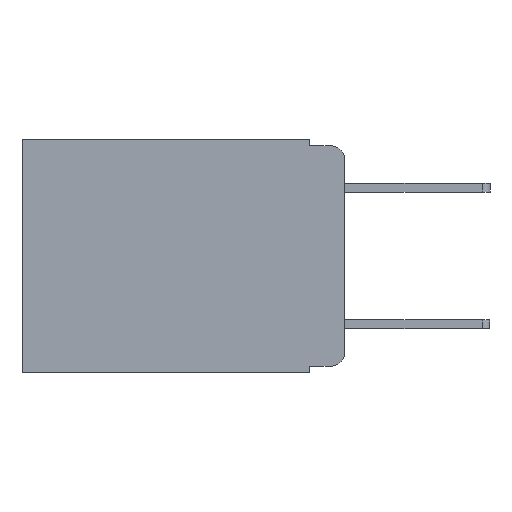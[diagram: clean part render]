
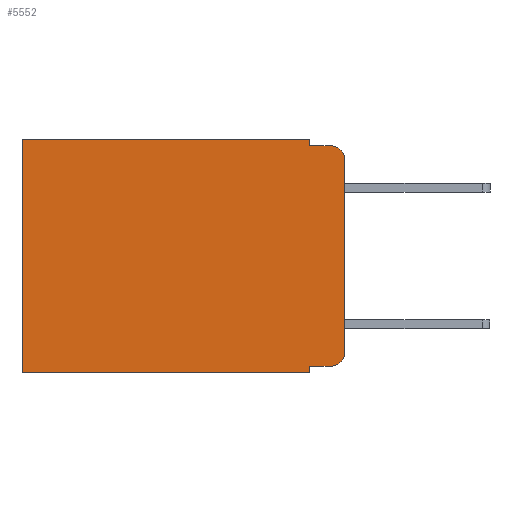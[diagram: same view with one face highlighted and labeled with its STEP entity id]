
A CAD part, left-side view. The second image highlights one B-rep face of the part: STEP entity #5552.
In plain terms, the highlighted planar face has unit normal (-1, 0, 0).
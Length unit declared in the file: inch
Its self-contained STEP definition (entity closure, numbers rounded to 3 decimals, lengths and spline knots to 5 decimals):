
#8 = VECTOR ( 'NONE', #10532, 39.37008 ) ;
#55 = CARTESIAN_POINT ( 'NONE',  ( 0.298, 0., 0. ) ) ;
#205 = LINE ( 'NONE', #9611, #5997 ) ;
#287 = ORIENTED_EDGE ( 'NONE', *, *, #2690, .F. ) ;
#311 = CARTESIAN_POINT ( 'NONE',  ( 0.298, 0.02, -0.333 ) ) ;
#372 = VECTOR ( 'NONE', #2864, 39.37008 ) ;
#613 = VERTEX_POINT ( 'NONE', #10655 ) ;
#626 = ORIENTED_EDGE ( 'NONE', *, *, #2716, .T. ) ;
#729 = CARTESIAN_POINT ( 'NONE',  ( 0.298, 0.473, 0. ) ) ;
#825 = ORIENTED_EDGE ( 'NONE', *, *, #6693, .T. ) ;
#1047 = LINE ( 'NONE', #729, #372 ) ;
#1069 = VERTEX_POINT ( 'NONE', #9491 ) ;
#1205 = VECTOR ( 'NONE', #4207, 39.37008 ) ;
#1219 = DIRECTION ( 'NONE',  ( 1., 0., 0. ) ) ;
#1309 = AXIS2_PLACEMENT_3D ( 'NONE', #1734, #8865, #2820 ) ;
#1691 = ORIENTED_EDGE ( 'NONE', *, *, #2676, .F. ) ;
#1734 = CARTESIAN_POINT ( 'NONE',  ( 0.298, 0.02, -0.03 ) ) ;
#1859 = CARTESIAN_POINT ( 'NONE',  ( 0.298, 0., -0.03 ) ) ;
#1904 = ORIENTED_EDGE ( 'NONE', *, *, #8988, .F. ) ;
#2116 = ORIENTED_EDGE ( 'NONE', *, *, #6798, .F. ) ;
#2216 = EDGE_LOOP ( 'NONE', ( #1904, #2267, #287, #1691, #626, #825, #2370, #2116, #2641, #12103 ) ) ;
#2230 = VERTEX_POINT ( 'NONE', #11432 ) ;
#2267 = ORIENTED_EDGE ( 'NONE', *, *, #8161, .T. ) ;
#2370 = ORIENTED_EDGE ( 'NONE', *, *, #3287, .F. ) ;
#2606 = DIRECTION ( 'NONE',  ( 0., -1., 0. ) ) ;
#2641 = ORIENTED_EDGE ( 'NONE', *, *, #7131, .T. ) ;
#2676 = EDGE_CURVE ( 'NONE', #1069, #2230, #3109, .T. ) ;
#2690 = EDGE_CURVE ( 'NONE', #2230, #613, #11928, .T. ) ;
#2716 = EDGE_CURVE ( 'NONE', #1069, #6191, #8904, .T. ) ;
#2820 = DIRECTION ( 'NONE',  ( 0., 0., -1. ) ) ;
#2864 = DIRECTION ( 'NONE',  ( 0., 0., -1. ) ) ;
#3109 = LINE ( 'NONE', #11004, #4253 ) ;
#3244 = LINE ( 'NONE', #5622, #8 ) ;
#3287 = EDGE_CURVE ( 'NONE', #9546, #12677, #205, .T. ) ;
#3580 = VECTOR ( 'NONE', #7004, 39.37008 ) ;
#3640 = VERTEX_POINT ( 'NONE', #10193 ) ;
#3723 = CARTESIAN_POINT ( 'NONE',  ( 0.298, 0.02, -0.313 ) ) ;
#4207 = DIRECTION ( 'NONE',  ( 0., 0., -1. ) ) ;
#4253 = VECTOR ( 'NONE', #11816, 39.37008 ) ;
#4535 = VECTOR ( 'NONE', #8374, 39.37008 ) ;
#4757 = DIRECTION ( 'NONE',  ( 0., 0., -1. ) ) ;
#4886 = CARTESIAN_POINT ( 'NONE',  ( 0.298, 0.473, 0. ) ) ;
#5406 = VERTEX_POINT ( 'NONE', #1859 ) ;
#5552 = ADVANCED_FACE ( 'NONE', ( #11797 ), #6470, .F. ) ;
#5622 = CARTESIAN_POINT ( 'NONE',  ( 0.298, 0.051, -0.333 ) ) ;
#5997 = VECTOR ( 'NONE', #7554, 39.37008 ) ;
#6014 = CIRCLE ( 'NONE', #1309, 0.02 ) ;
#6073 = CARTESIAN_POINT ( 'NONE',  ( 0.298, 0.051, -0.333 ) ) ;
#6191 = VERTEX_POINT ( 'NONE', #4886 ) ;
#6244 = VERTEX_POINT ( 'NONE', #6073 ) ;
#6470 = PLANE ( 'NONE',  #9592 ) ;
#6479 = CARTESIAN_POINT ( 'NONE',  ( 0.298, 0.473, -0.343 ) ) ;
#6617 = VECTOR ( 'NONE', #2606, 39.37008 ) ;
#6693 = EDGE_CURVE ( 'NONE', #6191, #12677, #1047, .T. ) ;
#6798 = EDGE_CURVE ( 'NONE', #6244, #9546, #9372, .T. ) ;
#7004 = DIRECTION ( 'NONE',  ( 0., 1., 0. ) ) ;
#7131 = EDGE_CURVE ( 'NONE', #6244, #9691, #3244, .T. ) ;
#7224 = LINE ( 'NONE', #55, #4535 ) ;
#7461 = CARTESIAN_POINT ( 'NONE',  ( 0.298, 0., 0. ) ) ;
#7484 = EDGE_CURVE ( 'NONE', #9691, #3640, #12308, .T. ) ;
#7554 = DIRECTION ( 'NONE',  ( 0., 1., 0. ) ) ;
#8156 = CARTESIAN_POINT ( 'NONE',  ( 0.298, 0.051, 0. ) ) ;
#8161 = EDGE_CURVE ( 'NONE', #5406, #613, #6014, .T. ) ;
#8374 = DIRECTION ( 'NONE',  ( 0., 0., -1. ) ) ;
#8436 = DIRECTION ( 'NONE',  ( 0., 0., -1. ) ) ;
#8865 = DIRECTION ( 'NONE',  ( -1., 0., 0. ) ) ;
#8904 = LINE ( 'NONE', #12608, #3580 ) ;
#8988 = EDGE_CURVE ( 'NONE', #5406, #3640, #7224, .T. ) ;
#9372 = LINE ( 'NONE', #8156, #1205 ) ;
#9491 = CARTESIAN_POINT ( 'NONE',  ( 0.298, 0.051, 0. ) ) ;
#9546 = VERTEX_POINT ( 'NONE', #10325 ) ;
#9592 = AXIS2_PLACEMENT_3D ( 'NONE', #7461, #1219, #8436 ) ;
#9603 = AXIS2_PLACEMENT_3D ( 'NONE', #3723, #10593, #4757 ) ;
#9611 = CARTESIAN_POINT ( 'NONE',  ( 0.298, 0., -0.343 ) ) ;
#9691 = VERTEX_POINT ( 'NONE', #311 ) ;
#10193 = CARTESIAN_POINT ( 'NONE',  ( 0.298, 0., -0.313 ) ) ;
#10325 = CARTESIAN_POINT ( 'NONE',  ( 0.298, 0.051, -0.343 ) ) ;
#10532 = DIRECTION ( 'NONE',  ( 0., -1., 0. ) ) ;
#10593 = DIRECTION ( 'NONE',  ( -1., 0., 0. ) ) ;
#10655 = CARTESIAN_POINT ( 'NONE',  ( 0.298, 0.02, -0.01 ) ) ;
#11004 = CARTESIAN_POINT ( 'NONE',  ( 0.298, 0.051, 0. ) ) ;
#11432 = CARTESIAN_POINT ( 'NONE',  ( 0.298, 0.051, -0.01 ) ) ;
#11748 = CARTESIAN_POINT ( 'NONE',  ( 0.298, 0.051, -0.01 ) ) ;
#11797 = FACE_OUTER_BOUND ( 'NONE', #2216, .T. ) ;
#11816 = DIRECTION ( 'NONE',  ( 0., 0., -1. ) ) ;
#11928 = LINE ( 'NONE', #11748, #6617 ) ;
#12103 = ORIENTED_EDGE ( 'NONE', *, *, #7484, .T. ) ;
#12308 = CIRCLE ( 'NONE', #9603, 0.02 ) ;
#12608 = CARTESIAN_POINT ( 'NONE',  ( 0.298, 0., 0. ) ) ;
#12677 = VERTEX_POINT ( 'NONE', #6479 ) ;
